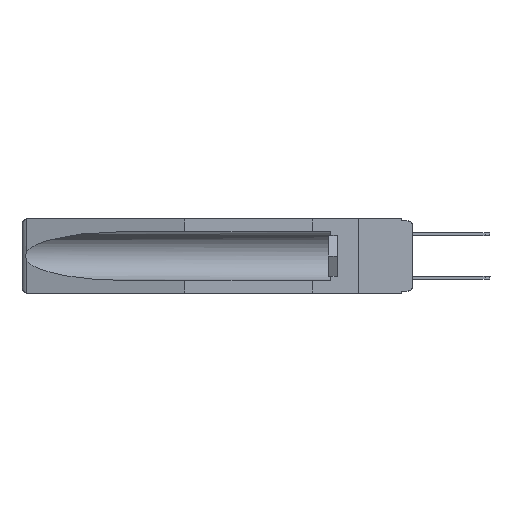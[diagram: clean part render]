
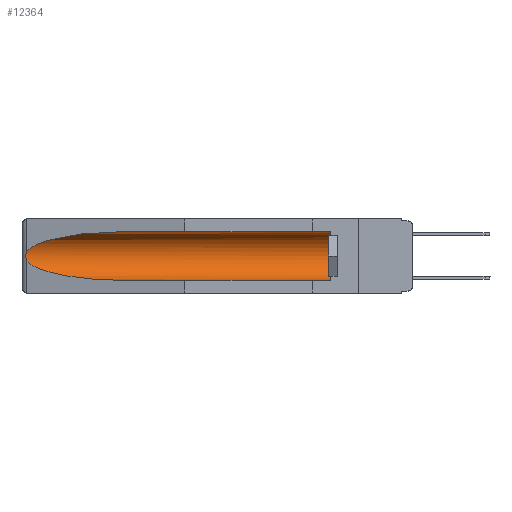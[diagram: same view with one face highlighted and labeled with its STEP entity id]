
A CAD part, left-side view. The second image highlights one B-rep face of the part: STEP entity #12364.
In plain terms, the highlighted cylindrical face has radius 2.857 mm (diameter 5.715 mm), a partial arc.
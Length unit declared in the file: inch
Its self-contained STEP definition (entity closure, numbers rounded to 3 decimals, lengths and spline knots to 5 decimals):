
#91 = FACE_OUTER_BOUND ( 'NONE', #1556, .T. ) ;
#685 = VERTEX_POINT ( 'NONE', #4071 ) ;
#1195 = DIRECTION ( 'NONE',  ( 0., 1., 0. ) ) ;
#1281 = VERTEX_POINT ( 'NONE', #10939 ) ;
#1406 = CARTESIAN_POINT ( 'NONE',  ( 0.155, 1.07973, -0.059 ) ) ;
#1556 = EDGE_LOOP ( 'NONE', ( #4764, #3935, #11532, #3134, #7590, #5713 ) ) ;
#1981 = CARTESIAN_POINT ( 'NONE',  ( 0.155, 0.126, -0.059 ) ) ;
#2375 = DIRECTION ( 'NONE',  ( 0., -1., 0. ) ) ;
#2760 = EDGE_CURVE ( 'NONE', #4003, #4949, #10648, .T. ) ;
#2861 = CYLINDRICAL_SURFACE ( 'NONE', #9848, 0.1125 ) ;
#2954 = DIRECTION ( 'NONE',  ( 0., 0., 1. ) ) ;
#3033 = CARTESIAN_POINT ( 'NONE',  ( 0.2675, 1.53308, -0.16763 ) ) ;
#3134 = ORIENTED_EDGE ( 'NONE', *, *, #14872, .F. ) ;
#3430 =( BOUNDED_CURVE ( )  B_SPLINE_CURVE ( 3, ( #9649, #18266, #12530, #7118 ),
 .UNSPECIFIED., .F., .T. ) 
 B_SPLINE_CURVE_WITH_KNOTS ( ( 4, 4 ),
 ( 0.1948, 1.5708 ),
 .UNSPECIFIED. ) 
 CURVE ( )  GEOMETRIC_REPRESENTATION_ITEM ( )  RATIONAL_B_SPLINE_CURVE ( ( 1., 0.848, 0.848, 1. ) ) 
 REPRESENTATION_ITEM ( '' )  );
#3935 = ORIENTED_EDGE ( 'NONE', *, *, #2760, .T. ) ;
#4003 = VERTEX_POINT ( 'NONE', #14126 ) ;
#4071 = CARTESIAN_POINT ( 'NONE',  ( 0.155, 1.07973, -0.284 ) ) ;
#4497 = CARTESIAN_POINT ( 'NONE',  ( 0.26655, 1.53094, -0.18657 ) ) ;
#4764 = ORIENTED_EDGE ( 'NONE', *, *, #13741, .T. ) ;
#4949 = VERTEX_POINT ( 'NONE', #13144 ) ;
#5205 =( BOUNDED_CURVE ( )  B_SPLINE_CURVE ( 3, ( #12647, #18290, #8725, #11155 ),
 .UNSPECIFIED., .F., .T. ) 
 B_SPLINE_CURVE_WITH_KNOTS ( ( 4, 4 ),
 ( 4.71239, 6.08839 ),
 .UNSPECIFIED. ) 
 CURVE ( )  GEOMETRIC_REPRESENTATION_ITEM ( )  RATIONAL_B_SPLINE_CURVE ( ( 1., 0.848, 0.848, 1. ) ) 
 REPRESENTATION_ITEM ( '' )  );
#5713 = ORIENTED_EDGE ( 'NONE', *, *, #11128, .T. ) ;
#6197 = CARTESIAN_POINT ( 'NONE',  ( 0.26597, 1.52961, -0.15275 ) ) ;
#6947 = CARTESIAN_POINT ( 'NONE',  ( 0.155, -0.30754, -0.1715 ) ) ;
#7118 = CARTESIAN_POINT ( 'NONE',  ( 0.155, 1.07973, -0.284 ) ) ;
#7590 = ORIENTED_EDGE ( 'NONE', *, *, #12749, .T. ) ;
#8414 = EDGE_CURVE ( 'NONE', #4949, #685, #3430, .T. ) ;
#8526 = LINE ( 'NONE', #13912, #11112 ) ;
#8725 = CARTESIAN_POINT ( 'NONE',  ( 0.25451, 1.48313, -0.09465 ) ) ;
#8991 = CARTESIAN_POINT ( 'NONE',  ( 0.26654, 1.53092, -0.15636 ) ) ;
#9554 = AXIS2_PLACEMENT_3D ( 'NONE', #10859, #2375, #13720 ) ;
#9649 = CARTESIAN_POINT ( 'NONE',  ( 0.26537, 1.52718, -0.19328 ) ) ;
#9848 = AXIS2_PLACEMENT_3D ( 'NONE', #6947, #12744, #2954 ) ;
#9927 = CARTESIAN_POINT ( 'NONE',  ( 0.155, -0.30754, -0.059 ) ) ;
#10132 = CARTESIAN_POINT ( 'NONE',  ( 0.26597, 1.5296, -0.19026 ) ) ;
#10460 = CIRCLE ( 'NONE', #9554, 0.1125 ) ;
#10648 = B_SPLINE_CURVE_WITH_KNOTS ( 'NONE', 3,
 ( #13359, #6197, #8991, #11610, #3033, #14467, #17531, #4497, #10132, #17262 ),
 .UNSPECIFIED., .F., .F.,
 ( 4, 2, 2, 2, 4 ),
 ( 0., 0.00029, 0.00058, 0.00087, 0.00117 ),
 .UNSPECIFIED. ) ;
#10706 = VERTEX_POINT ( 'NONE', #1406 ) ;
#10859 = CARTESIAN_POINT ( 'NONE',  ( 0.155, 0.126, -0.1715 ) ) ;
#10939 = CARTESIAN_POINT ( 'NONE',  ( 0.155, 0.126, -0.284 ) ) ;
#11112 = VECTOR ( 'NONE', #1195, 39.37008 ) ;
#11128 = EDGE_CURVE ( 'NONE', #17009, #10706, #16968, .T. ) ;
#11155 = CARTESIAN_POINT ( 'NONE',  ( 0.26537, 1.52718, -0.14972 ) ) ;
#11532 = ORIENTED_EDGE ( 'NONE', *, *, #8414, .T. ) ;
#11610 = CARTESIAN_POINT ( 'NONE',  ( 0.2673, 1.5327, -0.16383 ) ) ;
#12364 = ADVANCED_FACE ( 'NONE', ( #91 ), #2861, .F. ) ;
#12530 = CARTESIAN_POINT ( 'NONE',  ( 0.21114, 1.30732, -0.284 ) ) ;
#12647 = CARTESIAN_POINT ( 'NONE',  ( 0.155, 1.07973, -0.059 ) ) ;
#12744 = DIRECTION ( 'NONE',  ( 0., 1., 0. ) ) ;
#12749 = EDGE_CURVE ( 'NONE', #1281, #17009, #10460, .T. ) ;
#12899 = DIRECTION ( 'NONE',  ( 0., 1., 0. ) ) ;
#13144 = CARTESIAN_POINT ( 'NONE',  ( 0.26537, 1.52718, -0.19328 ) ) ;
#13359 = CARTESIAN_POINT ( 'NONE',  ( 0.26537, 1.52718, -0.14972 ) ) ;
#13720 = DIRECTION ( 'NONE',  ( 0., 0., 1. ) ) ;
#13741 = EDGE_CURVE ( 'NONE', #10706, #4003, #5205, .T. ) ;
#13912 = CARTESIAN_POINT ( 'NONE',  ( 0.155, -0.30754, -0.284 ) ) ;
#14126 = CARTESIAN_POINT ( 'NONE',  ( 0.26537, 1.52718, -0.14972 ) ) ;
#14467 = CARTESIAN_POINT ( 'NONE',  ( 0.2675, 1.53308, -0.17534 ) ) ;
#14872 = EDGE_CURVE ( 'NONE', #1281, #685, #8526, .T. ) ;
#16522 = VECTOR ( 'NONE', #12899, 39.37008 ) ;
#16968 = LINE ( 'NONE', #9927, #16522 ) ;
#17009 = VERTEX_POINT ( 'NONE', #1981 ) ;
#17262 = CARTESIAN_POINT ( 'NONE',  ( 0.26537, 1.52718, -0.19328 ) ) ;
#17531 = CARTESIAN_POINT ( 'NONE',  ( 0.2673, 1.53269, -0.17917 ) ) ;
#18266 = CARTESIAN_POINT ( 'NONE',  ( 0.25451, 1.48313, -0.24835 ) ) ;
#18290 = CARTESIAN_POINT ( 'NONE',  ( 0.21114, 1.30732, -0.059 ) ) ;
